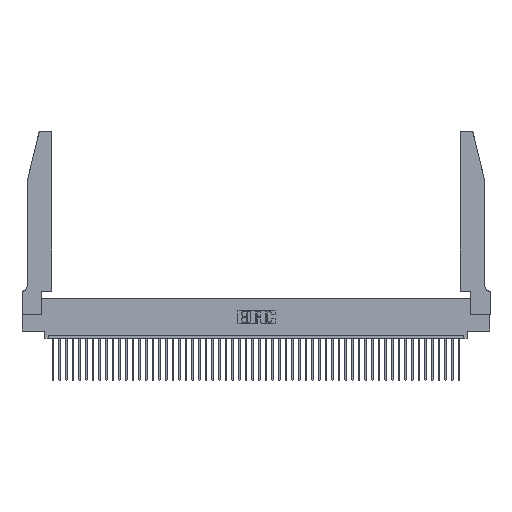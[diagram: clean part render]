
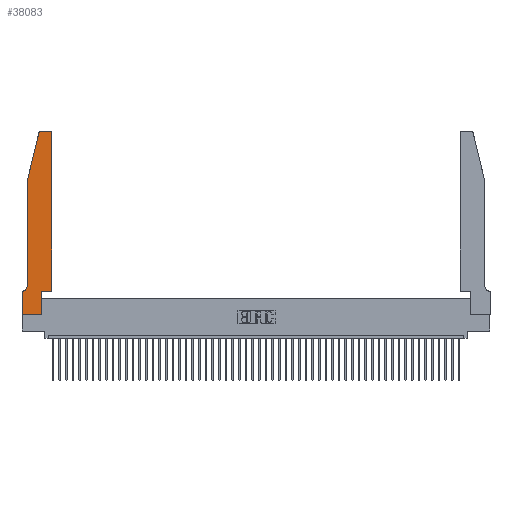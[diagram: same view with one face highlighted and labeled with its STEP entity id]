
A CAD part, top view. The second image highlights one B-rep face of the part: STEP entity #38083.
In plain terms, the highlighted planar face has unit normal (0, 0, 1).
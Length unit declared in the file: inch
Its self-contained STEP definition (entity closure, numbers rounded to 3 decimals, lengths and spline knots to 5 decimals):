
#410 = VECTOR ( 'NONE', #20295, 39.37008 ) ;
#435 = VECTOR ( 'NONE', #48652, 39.37008 ) ;
#516 = DIRECTION ( 'NONE',  ( -1., 0., 0. ) ) ;
#720 = ORIENTED_EDGE ( 'NONE', *, *, #8164, .T. ) ;
#1028 = LINE ( 'NONE', #14845, #17639 ) ;
#1186 = EDGE_LOOP ( 'NONE', ( #25747, #14611, #34468, #14489, #20885, #2900, #48095, #36842, #25544, #720, #3345, #28539 ) ) ;
#1609 = LINE ( 'NONE', #46836, #410 ) ;
#1678 = FACE_OUTER_BOUND ( 'NONE', #1186, .T. ) ;
#2900 = ORIENTED_EDGE ( 'NONE', *, *, #15553, .T. ) ;
#3345 = ORIENTED_EDGE ( 'NONE', *, *, #38936, .T. ) ;
#4119 = CARTESIAN_POINT ( 'NONE',  ( 0.0755, 2., 0.37 ) ) ;
#6158 = DIRECTION ( 'NONE',  ( 0., 0., 1. ) ) ;
#6537 = VERTEX_POINT ( 'NONE', #14981 ) ;
#6930 = VERTEX_POINT ( 'NONE', #25600 ) ;
#8164 = EDGE_CURVE ( 'NONE', #9634, #6537, #19014, .T. ) ;
#9334 = CARTESIAN_POINT ( 'NONE',  ( 0., 0., 0.37 ) ) ;
#9457 = CARTESIAN_POINT ( 'NONE',  ( 0.284, 2.75, 0.37 ) ) ;
#9460 = DIRECTION ( 'NONE',  ( 0., 0., -1. ) ) ;
#9579 = CARTESIAN_POINT ( 'NONE',  ( 0.4505, 2.72, 0.37 ) ) ;
#9634 = VERTEX_POINT ( 'NONE', #26497 ) ;
#10354 = VECTOR ( 'NONE', #34328, 39.37008 ) ;
#10575 = LINE ( 'NONE', #16907, #17036 ) ;
#11161 = EDGE_CURVE ( 'NONE', #27403, #17785, #1609, .T. ) ;
#11492 = EDGE_CURVE ( 'NONE', #46730, #45391, #36473, .T. ) ;
#12022 = EDGE_CURVE ( 'NONE', #17785, #9634, #22268, .T. ) ;
#12126 = CARTESIAN_POINT ( 'NONE',  ( 0.4505, 0.35, 0.37 ) ) ;
#12372 = CARTESIAN_POINT ( 'NONE',  ( 0.4205, 2.72, 0.37 ) ) ;
#13051 = DIRECTION ( 'NONE',  ( 1., 0., 0. ) ) ;
#14489 = ORIENTED_EDGE ( 'NONE', *, *, #46876, .T. ) ;
#14611 = ORIENTED_EDGE ( 'NONE', *, *, #31534, .T. ) ;
#14845 = CARTESIAN_POINT ( 'NONE',  ( 0.0755, 2., 0.37 ) ) ;
#14981 = CARTESIAN_POINT ( 'NONE',  ( 0.4505, 0.35, 0.37 ) ) ;
#15553 = EDGE_CURVE ( 'NONE', #6930, #17210, #29046, .T. ) ;
#15859 = CARTESIAN_POINT ( 'NONE',  ( 0.0055, 0.42, 0.37 ) ) ;
#16619 = CARTESIAN_POINT ( 'NONE',  ( 0.2865, 0.35, 0.37 ) ) ;
#16907 = CARTESIAN_POINT ( 'NONE',  ( 0.2605, 2.75, 0.37 ) ) ;
#17036 = VECTOR ( 'NONE', #47131, 39.37008 ) ;
#17210 = VERTEX_POINT ( 'NONE', #45594 ) ;
#17354 = EDGE_CURVE ( 'NONE', #45391, #48058, #10575, .T. ) ;
#17639 = VECTOR ( 'NONE', #26551, 39.37008 ) ;
#17785 = VERTEX_POINT ( 'NONE', #21686 ) ;
#17922 = DIRECTION ( 'NONE',  ( 1., 0., 0. ) ) ;
#18744 = VERTEX_POINT ( 'NONE', #27753 ) ;
#19014 = LINE ( 'NONE', #24259, #27865 ) ;
#20015 = DIRECTION ( 'NONE',  ( 0., 0., 1. ) ) ;
#20295 = DIRECTION ( 'NONE',  ( 1., 0., 0. ) ) ;
#20433 = CIRCLE ( 'NONE', #24646, 0.03 ) ;
#20885 = ORIENTED_EDGE ( 'NONE', *, *, #36446, .T. ) ;
#21595 = CARTESIAN_POINT ( 'NONE',  ( 0.0755, 0.35, 0.37 ) ) ;
#21686 = CARTESIAN_POINT ( 'NONE',  ( 0.2865, 0., 0.37 ) ) ;
#22268 = LINE ( 'NONE', #16619, #32882 ) ;
#22540 = LINE ( 'NONE', #33387, #23030 ) ;
#22558 = CIRCLE ( 'NONE', #37116, 0.07 ) ;
#23030 = VECTOR ( 'NONE', #41136, 39.37008 ) ;
#24259 = CARTESIAN_POINT ( 'NONE',  ( 0.4505, 0.35, 0.37 ) ) ;
#24646 = AXIS2_PLACEMENT_3D ( 'NONE', #33091, #33408, #17922 ) ;
#25481 = VECTOR ( 'NONE', #33260, 39.37008 ) ;
#25544 = ORIENTED_EDGE ( 'NONE', *, *, #12022, .T. ) ;
#25591 = EDGE_CURVE ( 'NONE', #17210, #27403, #27645, .T. ) ;
#25600 = CARTESIAN_POINT ( 'NONE',  ( 0.0055, 0.35, 0.37 ) ) ;
#25747 = ORIENTED_EDGE ( 'NONE', *, *, #17354, .T. ) ;
#26497 = CARTESIAN_POINT ( 'NONE',  ( 0.2865, 0.35, 0.37 ) ) ;
#26551 = DIRECTION ( 'NONE',  ( -0.239, -0.971, 0. ) ) ;
#26944 = DIRECTION ( 'NONE',  ( 1., 0., 0. ) ) ;
#27403 = VERTEX_POINT ( 'NONE', #31804 ) ;
#27645 = LINE ( 'NONE', #9334, #435 ) ;
#27753 = CARTESIAN_POINT ( 'NONE',  ( 0.25487, 2.72718, 0.37 ) ) ;
#27865 = VECTOR ( 'NONE', #39944, 39.37008 ) ;
#28539 = ORIENTED_EDGE ( 'NONE', *, *, #11492, .T. ) ;
#29046 = LINE ( 'NONE', #21595, #25481 ) ;
#30304 = EDGE_CURVE ( 'NONE', #18744, #47080, #1028, .T. ) ;
#31534 = EDGE_CURVE ( 'NONE', #48058, #18744, #20433, .T. ) ;
#31804 = CARTESIAN_POINT ( 'NONE',  ( 0., 0., 0.37 ) ) ;
#32882 = VECTOR ( 'NONE', #46472, 39.37008 ) ;
#33091 = CARTESIAN_POINT ( 'NONE',  ( 0.284, 2.72, 0.37 ) ) ;
#33260 = DIRECTION ( 'NONE',  ( -1., 0., 0. ) ) ;
#33387 = CARTESIAN_POINT ( 'NONE',  ( 0.0755, 2., 0.37 ) ) ;
#33408 = DIRECTION ( 'NONE',  ( 0., 0., 1. ) ) ;
#34328 = DIRECTION ( 'NONE',  ( 0., 1., 0. ) ) ;
#34468 = ORIENTED_EDGE ( 'NONE', *, *, #30304, .T. ) ;
#34861 = CARTESIAN_POINT ( 'NONE',  ( 0.0755, 0.42, 0.37 ) ) ;
#36446 = EDGE_CURVE ( 'NONE', #43638, #6930, #22558, .T. ) ;
#36473 = CIRCLE ( 'NONE', #45738, 0.03 ) ;
#36842 = ORIENTED_EDGE ( 'NONE', *, *, #11161, .T. ) ;
#37116 = AXIS2_PLACEMENT_3D ( 'NONE', #15859, #9460, #516 ) ;
#38083 = ADVANCED_FACE ( 'NONE', ( #1678 ), #47410, .T. ) ;
#38936 = EDGE_CURVE ( 'NONE', #6537, #46730, #48179, .T. ) ;
#39944 = DIRECTION ( 'NONE',  ( 1., 0., 0. ) ) ;
#41136 = DIRECTION ( 'NONE',  ( 0., -1., 0. ) ) ;
#43638 = VERTEX_POINT ( 'NONE', #34861 ) ;
#44092 = AXIS2_PLACEMENT_3D ( 'NONE', #47585, #6158, #13051 ) ;
#45391 = VERTEX_POINT ( 'NONE', #48643 ) ;
#45594 = CARTESIAN_POINT ( 'NONE',  ( 0., 0.35, 0.37 ) ) ;
#45738 = AXIS2_PLACEMENT_3D ( 'NONE', #12372, #20015, #26944 ) ;
#46472 = DIRECTION ( 'NONE',  ( 0., 1., 0. ) ) ;
#46730 = VERTEX_POINT ( 'NONE', #9579 ) ;
#46836 = CARTESIAN_POINT ( 'NONE',  ( 0., 0., 0.37 ) ) ;
#46876 = EDGE_CURVE ( 'NONE', #47080, #43638, #22540, .T. ) ;
#47080 = VERTEX_POINT ( 'NONE', #4119 ) ;
#47131 = DIRECTION ( 'NONE',  ( -1., 0., 0. ) ) ;
#47410 = PLANE ( 'NONE',  #44092 ) ;
#47585 = CARTESIAN_POINT ( 'NONE',  ( 0., 0.35, 0.37 ) ) ;
#48058 = VERTEX_POINT ( 'NONE', #9457 ) ;
#48095 = ORIENTED_EDGE ( 'NONE', *, *, #25591, .T. ) ;
#48179 = LINE ( 'NONE', #12126, #10354 ) ;
#48643 = CARTESIAN_POINT ( 'NONE',  ( 0.4205, 2.75, 0.37 ) ) ;
#48652 = DIRECTION ( 'NONE',  ( 0., -1., 0. ) ) ;
